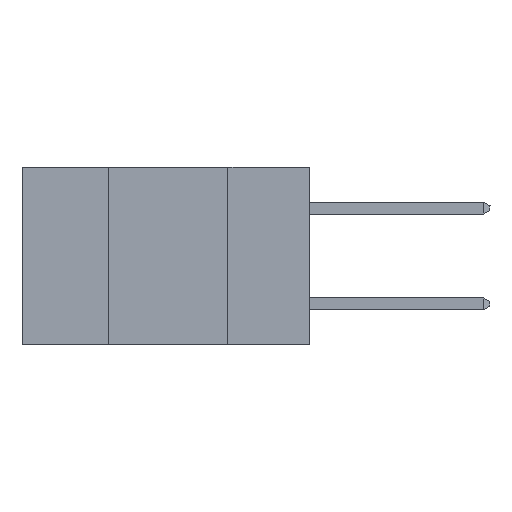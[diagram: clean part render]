
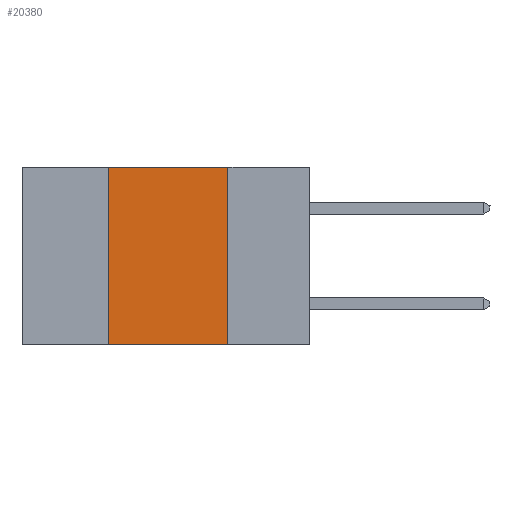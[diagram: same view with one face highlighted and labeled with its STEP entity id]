
A CAD part, left-side view. The second image highlights one B-rep face of the part: STEP entity #20380.
In plain terms, the highlighted planar face has unit normal (-1, 0, 0).
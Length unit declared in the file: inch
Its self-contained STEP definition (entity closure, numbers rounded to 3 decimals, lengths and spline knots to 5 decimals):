
#1052 = LINE ( 'NONE', #6757, #21359 ) ;
#1171 = CARTESIAN_POINT ( 'NONE',  ( 0., 0.6, 0. ) ) ;
#1669 = CARTESIAN_POINT ( 'NONE',  ( 0., 0.42, 0. ) ) ;
#1861 = DIRECTION ( 'NONE',  ( 0., 0., -1. ) ) ;
#2084 = ORIENTED_EDGE ( 'NONE', *, *, #2280, .F. ) ;
#2280 = EDGE_CURVE ( 'NONE', #5473, #5736, #19227, .T. ) ;
#2660 = DIRECTION ( 'NONE',  ( 0., -1., 0. ) ) ;
#3744 = ORIENTED_EDGE ( 'NONE', *, *, #8630, .F. ) ;
#4037 = VECTOR ( 'NONE', #16020, 39.37008 ) ;
#4894 = LINE ( 'NONE', #1171, #4037 ) ;
#5473 = VERTEX_POINT ( 'NONE', #12237 ) ;
#5736 = VERTEX_POINT ( 'NONE', #16894 ) ;
#6268 = CARTESIAN_POINT ( 'NONE',  ( 0., 0.17, 0. ) ) ;
#6352 = ORIENTED_EDGE ( 'NONE', *, *, #15321, .F. ) ;
#6539 = AXIS2_PLACEMENT_3D ( 'NONE', #7703, #18928, #1861 ) ;
#6757 = CARTESIAN_POINT ( 'NONE',  ( 0., 0.6, -0.37 ) ) ;
#6982 = EDGE_LOOP ( 'NONE', ( #2084, #6352, #3744, #20676 ) ) ;
#7148 = CARTESIAN_POINT ( 'NONE',  ( 0., 0.42, 0. ) ) ;
#7514 = DIRECTION ( 'NONE',  ( 0., 0., 1. ) ) ;
#7703 = CARTESIAN_POINT ( 'NONE',  ( 0., 0.6, 0. ) ) ;
#8630 = EDGE_CURVE ( 'NONE', #18125, #16735, #14918, .T. ) ;
#11125 = VECTOR ( 'NONE', #15532, 39.37008 ) ;
#11397 = PLANE ( 'NONE',  #6539 ) ;
#12078 = EDGE_CURVE ( 'NONE', #18125, #5736, #1052, .T. ) ;
#12237 = CARTESIAN_POINT ( 'NONE',  ( 0., 0.17, 0. ) ) ;
#12970 = VECTOR ( 'NONE', #7514, 39.37008 ) ;
#14907 = CARTESIAN_POINT ( 'NONE',  ( 0., 0.42, -0.37 ) ) ;
#14918 = LINE ( 'NONE', #7148, #12970 ) ;
#15107 = FACE_OUTER_BOUND ( 'NONE', #6982, .T. ) ;
#15321 = EDGE_CURVE ( 'NONE', #16735, #5473, #4894, .T. ) ;
#15532 = DIRECTION ( 'NONE',  ( 0., 0., -1. ) ) ;
#16020 = DIRECTION ( 'NONE',  ( 0., -1., 0. ) ) ;
#16735 = VERTEX_POINT ( 'NONE', #1669 ) ;
#16894 = CARTESIAN_POINT ( 'NONE',  ( 0., 0.17, -0.37 ) ) ;
#18125 = VERTEX_POINT ( 'NONE', #14907 ) ;
#18928 = DIRECTION ( 'NONE',  ( 1., 0., 0. ) ) ;
#19227 = LINE ( 'NONE', #6268, #11125 ) ;
#20380 = ADVANCED_FACE ( 'NONE', ( #15107 ), #11397, .F. ) ;
#20676 = ORIENTED_EDGE ( 'NONE', *, *, #12078, .T. ) ;
#21359 = VECTOR ( 'NONE', #2660, 39.37008 ) ;
